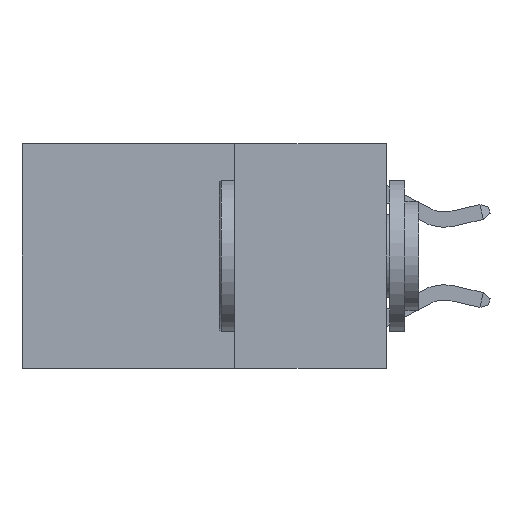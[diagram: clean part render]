
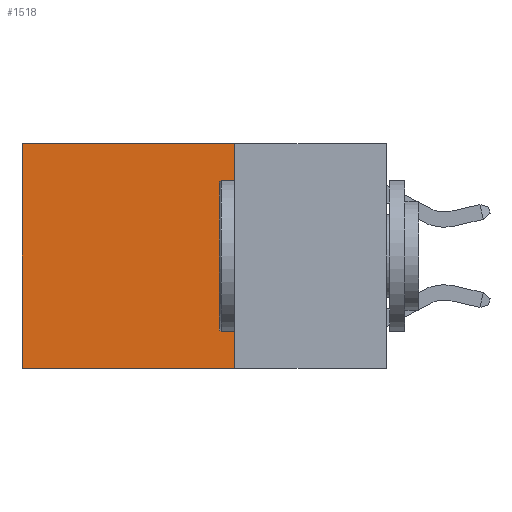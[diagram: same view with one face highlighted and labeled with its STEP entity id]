
A CAD part, left-side view. The second image highlights one B-rep face of the part: STEP entity #1518.
In plain terms, the highlighted planar face has unit normal (-1, 0, 0).
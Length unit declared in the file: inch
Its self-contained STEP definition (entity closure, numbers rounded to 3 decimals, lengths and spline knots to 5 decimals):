
#161 = CARTESIAN_POINT ( 'NONE',  ( 0.2625, 0.6, 0. ) ) ;
#432 = AXIS2_PLACEMENT_3D ( 'NONE', #7691, #3654, #10430 ) ;
#755 = FACE_OUTER_BOUND ( 'NONE', #11089, .T. ) ;
#1518 = ADVANCED_FACE ( 'NONE', ( #755 ), #12732, .F. ) ;
#1530 = VERTEX_POINT ( 'NONE', #29131 ) ;
#2394 = ORIENTED_EDGE ( 'NONE', *, *, #20632, .F. ) ;
#2993 = LINE ( 'NONE', #7158, #10730 ) ;
#3133 = VECTOR ( 'NONE', #21477, 39.37008 ) ;
#3654 = DIRECTION ( 'NONE',  ( 1., 0., 0. ) ) ;
#3682 = CARTESIAN_POINT ( 'NONE',  ( 0.2625, 0.25, 0. ) ) ;
#7158 = CARTESIAN_POINT ( 'NONE',  ( 0.2625, 0.25, 0. ) ) ;
#7518 = DIRECTION ( 'NONE',  ( 0., 0., -1. ) ) ;
#7691 = CARTESIAN_POINT ( 'NONE',  ( 0.2625, 0.25, 0. ) ) ;
#8385 = EDGE_CURVE ( 'NONE', #13548, #28723, #2993, .T. ) ;
#8415 = ORIENTED_EDGE ( 'NONE', *, *, #25800, .T. ) ;
#9028 = CARTESIAN_POINT ( 'NONE',  ( 0.2625, 0.25, -0.37 ) ) ;
#10430 = DIRECTION ( 'NONE',  ( 0., 0., -1. ) ) ;
#10527 = CARTESIAN_POINT ( 'NONE',  ( 0.2625, 0.6, 0. ) ) ;
#10730 = VECTOR ( 'NONE', #14524, 39.37008 ) ;
#11089 = EDGE_LOOP ( 'NONE', ( #8415, #2394, #27425, #22422 ) ) ;
#12732 = PLANE ( 'NONE',  #432 ) ;
#13548 = VERTEX_POINT ( 'NONE', #3682 ) ;
#14524 = DIRECTION ( 'NONE',  ( 0., 1., 0. ) ) ;
#15582 = VECTOR ( 'NONE', #29861, 39.37008 ) ;
#16867 = LINE ( 'NONE', #161, #3133 ) ;
#17879 = EDGE_CURVE ( 'NONE', #13548, #20723, #21458, .T. ) ;
#18506 = CARTESIAN_POINT ( 'NONE',  ( 0.2625, 0.25, -0.37 ) ) ;
#18854 = CARTESIAN_POINT ( 'NONE',  ( 0.2625, 0.25, 0. ) ) ;
#20507 = LINE ( 'NONE', #18506, #15582 ) ;
#20632 = EDGE_CURVE ( 'NONE', #20723, #1530, #20507, .T. ) ;
#20723 = VERTEX_POINT ( 'NONE', #9028 ) ;
#21458 = LINE ( 'NONE', #18854, #26688 ) ;
#21477 = DIRECTION ( 'NONE',  ( 0., 0., -1. ) ) ;
#22422 = ORIENTED_EDGE ( 'NONE', *, *, #8385, .T. ) ;
#25800 = EDGE_CURVE ( 'NONE', #28723, #1530, #16867, .T. ) ;
#26688 = VECTOR ( 'NONE', #7518, 39.37008 ) ;
#27425 = ORIENTED_EDGE ( 'NONE', *, *, #17879, .F. ) ;
#28723 = VERTEX_POINT ( 'NONE', #10527 ) ;
#29131 = CARTESIAN_POINT ( 'NONE',  ( 0.2625, 0.6, -0.37 ) ) ;
#29861 = DIRECTION ( 'NONE',  ( 0., 1., 0. ) ) ;
